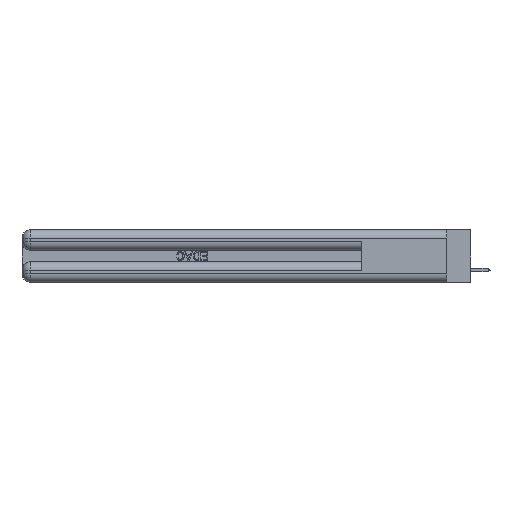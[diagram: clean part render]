
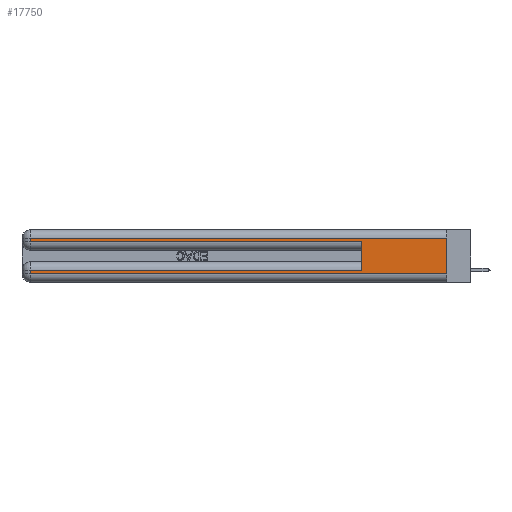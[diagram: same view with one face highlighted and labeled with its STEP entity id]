
A CAD part, left-side view. The second image highlights one B-rep face of the part: STEP entity #17750.
In plain terms, the highlighted planar face has unit normal (-1, 0, 0).
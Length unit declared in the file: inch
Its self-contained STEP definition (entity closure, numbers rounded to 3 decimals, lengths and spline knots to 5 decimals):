
#974 = LINE ( 'NONE', #44763, #3801 ) ;
#1086 = CARTESIAN_POINT ( 'NONE',  ( 0., 0., 0.285 ) ) ;
#1250 = DIRECTION ( 'NONE',  ( 0., -1., 0. ) ) ;
#1638 = CARTESIAN_POINT ( 'NONE',  ( 0., 2.94, 0.06 ) ) ;
#1704 = VERTEX_POINT ( 'NONE', #9113 ) ;
#3801 = VECTOR ( 'NONE', #16369, 39.37008 ) ;
#4507 = VERTEX_POINT ( 'NONE', #21429 ) ;
#6170 = FACE_OUTER_BOUND ( 'NONE', #28659, .T. ) ;
#7933 = CARTESIAN_POINT ( 'NONE',  ( 0., 0., 0.31 ) ) ;
#8088 = DIRECTION ( 'NONE',  ( 0., 1., 0. ) ) ;
#8621 = PLANE ( 'NONE',  #26202 ) ;
#8709 = DIRECTION ( 'NONE',  ( 0., 1., 0. ) ) ;
#9016 = CARTESIAN_POINT ( 'NONE',  ( 0., 0., 0.06 ) ) ;
#9112 = ORIENTED_EDGE ( 'NONE', *, *, #34354, .T. ) ;
#9113 = CARTESIAN_POINT ( 'NONE',  ( 0., 0.6, 0.285 ) ) ;
#9477 = VERTEX_POINT ( 'NONE', #9016 ) ;
#11796 = ORIENTED_EDGE ( 'NONE', *, *, #14431, .T. ) ;
#12272 = EDGE_CURVE ( 'NONE', #4507, #17944, #32030, .T. ) ;
#12353 = DIRECTION ( 'NONE',  ( 0., 0., -1. ) ) ;
#13986 = VERTEX_POINT ( 'NONE', #30331 ) ;
#14417 = DIRECTION ( 'NONE',  ( 0., 0., 1. ) ) ;
#14431 = EDGE_CURVE ( 'NONE', #39491, #9477, #27275, .T. ) ;
#14522 = DIRECTION ( 'NONE',  ( 0., -1., 0. ) ) ;
#14658 = ORIENTED_EDGE ( 'NONE', *, *, #42050, .T. ) ;
#14966 = LINE ( 'NONE', #7933, #27862 ) ;
#15528 = VECTOR ( 'NONE', #1250, 39.37008 ) ;
#16369 = DIRECTION ( 'NONE',  ( 0., 0., -1. ) ) ;
#17750 = ADVANCED_FACE ( 'NONE', ( #6170 ), #8621, .F. ) ;
#17860 = EDGE_CURVE ( 'NONE', #35505, #4507, #14966, .T. ) ;
#17944 = VERTEX_POINT ( 'NONE', #19724 ) ;
#18470 = EDGE_CURVE ( 'NONE', #34731, #39491, #974, .T. ) ;
#19416 = LINE ( 'NONE', #29465, #45164 ) ;
#19724 = CARTESIAN_POINT ( 'NONE',  ( 0., 2.94, 0.285 ) ) ;
#20671 = ORIENTED_EDGE ( 'NONE', *, *, #12272, .T. ) ;
#21429 = CARTESIAN_POINT ( 'NONE',  ( 0., 2.94, 0.31 ) ) ;
#22074 = ORIENTED_EDGE ( 'NONE', *, *, #18470, .T. ) ;
#22452 = VECTOR ( 'NONE', #12353, 39.37008 ) ;
#23832 = EDGE_CURVE ( 'NONE', #13986, #1704, #43364, .T. ) ;
#25036 = LINE ( 'NONE', #1086, #15528 ) ;
#26202 = AXIS2_PLACEMENT_3D ( 'NONE', #43548, #35869, #28501 ) ;
#27275 = LINE ( 'NONE', #34876, #33426 ) ;
#27559 = LINE ( 'NONE', #36292, #33701 ) ;
#27862 = VECTOR ( 'NONE', #8088, 39.37008 ) ;
#28501 = DIRECTION ( 'NONE',  ( 0., 0., -1. ) ) ;
#28659 = EDGE_LOOP ( 'NONE', ( #40639, #43538, #20671, #14658, #45945, #9112, #22074, #11796 ) ) ;
#29465 = CARTESIAN_POINT ( 'NONE',  ( 0., 0., 0.37 ) ) ;
#30331 = CARTESIAN_POINT ( 'NONE',  ( 0., 0.6, 0.085 ) ) ;
#30572 = DIRECTION ( 'NONE',  ( 0., 0., -1. ) ) ;
#30577 = CARTESIAN_POINT ( 'NONE',  ( 0., 2.94, 0.37 ) ) ;
#32030 = LINE ( 'NONE', #30577, #22452 ) ;
#32248 = CARTESIAN_POINT ( 'NONE',  ( 0., 0.6, 0.145 ) ) ;
#33426 = VECTOR ( 'NONE', #14522, 39.37008 ) ;
#33701 = VECTOR ( 'NONE', #8709, 39.37008 ) ;
#34354 = EDGE_CURVE ( 'NONE', #13986, #34731, #27559, .T. ) ;
#34731 = VERTEX_POINT ( 'NONE', #45792 ) ;
#34876 = CARTESIAN_POINT ( 'NONE',  ( 0., 0., 0.06 ) ) ;
#35505 = VERTEX_POINT ( 'NONE', #44117 ) ;
#35869 = DIRECTION ( 'NONE',  ( 1., 0., 0. ) ) ;
#36292 = CARTESIAN_POINT ( 'NONE',  ( 0., 0., 0.085 ) ) ;
#39491 = VERTEX_POINT ( 'NONE', #1638 ) ;
#40026 = VECTOR ( 'NONE', #14417, 39.37008 ) ;
#40639 = ORIENTED_EDGE ( 'NONE', *, *, #41989, .F. ) ;
#41989 = EDGE_CURVE ( 'NONE', #35505, #9477, #19416, .T. ) ;
#42050 = EDGE_CURVE ( 'NONE', #17944, #1704, #25036, .T. ) ;
#43364 = LINE ( 'NONE', #32248, #40026 ) ;
#43538 = ORIENTED_EDGE ( 'NONE', *, *, #17860, .T. ) ;
#43548 = CARTESIAN_POINT ( 'NONE',  ( 0., 0., 0.37 ) ) ;
#44117 = CARTESIAN_POINT ( 'NONE',  ( 0., 0., 0.31 ) ) ;
#44763 = CARTESIAN_POINT ( 'NONE',  ( 0., 2.94, 0.37 ) ) ;
#45164 = VECTOR ( 'NONE', #30572, 39.37008 ) ;
#45792 = CARTESIAN_POINT ( 'NONE',  ( 0., 2.94, 0.085 ) ) ;
#45945 = ORIENTED_EDGE ( 'NONE', *, *, #23832, .F. ) ;
